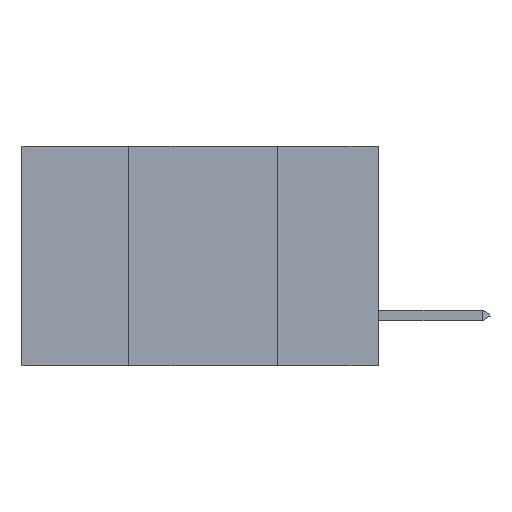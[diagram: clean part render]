
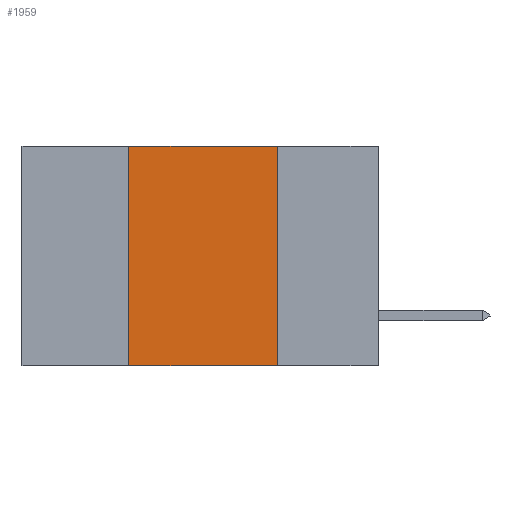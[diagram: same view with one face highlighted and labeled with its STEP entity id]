
A CAD part, left-side view. The second image highlights one B-rep face of the part: STEP entity #1959.
In plain terms, the highlighted planar face has unit normal (-1, 0, 0).
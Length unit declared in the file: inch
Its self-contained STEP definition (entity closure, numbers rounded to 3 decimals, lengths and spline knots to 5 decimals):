
#390 = DIRECTION ( 'NONE',  ( 0., 0., 1. ) ) ;
#544 = VECTOR ( 'NONE', #2401, 39.37008 ) ;
#747 = VERTEX_POINT ( 'NONE', #12343 ) ;
#1059 = LINE ( 'NONE', #7087, #5815 ) ;
#1959 = ADVANCED_FACE ( 'NONE', ( #2381 ), #11902, .F. ) ;
#2381 = FACE_OUTER_BOUND ( 'NONE', #11319, .T. ) ;
#2401 = DIRECTION ( 'NONE',  ( 0., 0., -1. ) ) ;
#2690 = EDGE_CURVE ( 'NONE', #8558, #747, #1059, .T. ) ;
#2816 = EDGE_CURVE ( 'NONE', #747, #8052, #12154, .T. ) ;
#3665 = ORIENTED_EDGE ( 'NONE', *, *, #2816, .F. ) ;
#3767 = CARTESIAN_POINT ( 'NONE',  ( 0., 0.17, -0.37 ) ) ;
#4620 = ORIENTED_EDGE ( 'NONE', *, *, #6682, .T. ) ;
#4641 = LINE ( 'NONE', #8347, #9450 ) ;
#4935 = AXIS2_PLACEMENT_3D ( 'NONE', #8965, #10903, #7131 ) ;
#5005 = LINE ( 'NONE', #8255, #544 ) ;
#5096 = EDGE_CURVE ( 'NONE', #8052, #11699, #5005, .T. ) ;
#5633 = CARTESIAN_POINT ( 'NONE',  ( 0., 0.17, 0. ) ) ;
#5815 = VECTOR ( 'NONE', #390, 39.37008 ) ;
#6163 = DIRECTION ( 'NONE',  ( 0., -1., 0. ) ) ;
#6682 = EDGE_CURVE ( 'NONE', #8558, #11699, #4641, .T. ) ;
#7087 = CARTESIAN_POINT ( 'NONE',  ( 0., 0.42, 0. ) ) ;
#7131 = DIRECTION ( 'NONE',  ( 0., 0., -1. ) ) ;
#8052 = VERTEX_POINT ( 'NONE', #5633 ) ;
#8255 = CARTESIAN_POINT ( 'NONE',  ( 0., 0.17, 0. ) ) ;
#8347 = CARTESIAN_POINT ( 'NONE',  ( 0., 0.6, -0.37 ) ) ;
#8370 = ORIENTED_EDGE ( 'NONE', *, *, #5096, .F. ) ;
#8558 = VERTEX_POINT ( 'NONE', #12305 ) ;
#8965 = CARTESIAN_POINT ( 'NONE',  ( 0., 0.6, 0. ) ) ;
#9450 = VECTOR ( 'NONE', #6163, 39.37008 ) ;
#10130 = CARTESIAN_POINT ( 'NONE',  ( 0., 0.6, 0. ) ) ;
#10211 = DIRECTION ( 'NONE',  ( 0., -1., 0. ) ) ;
#10469 = VECTOR ( 'NONE', #10211, 39.37008 ) ;
#10903 = DIRECTION ( 'NONE',  ( 1., 0., 0. ) ) ;
#11319 = EDGE_LOOP ( 'NONE', ( #8370, #3665, #11553, #4620 ) ) ;
#11553 = ORIENTED_EDGE ( 'NONE', *, *, #2690, .F. ) ;
#11699 = VERTEX_POINT ( 'NONE', #3767 ) ;
#11902 = PLANE ( 'NONE',  #4935 ) ;
#12154 = LINE ( 'NONE', #10130, #10469 ) ;
#12305 = CARTESIAN_POINT ( 'NONE',  ( 0., 0.42, -0.37 ) ) ;
#12343 = CARTESIAN_POINT ( 'NONE',  ( 0., 0.42, 0. ) ) ;
